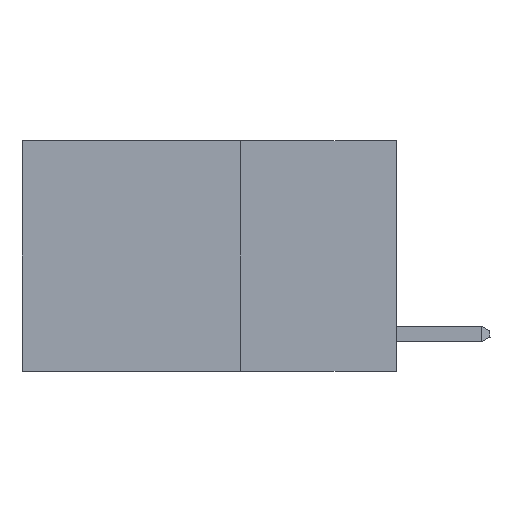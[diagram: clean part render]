
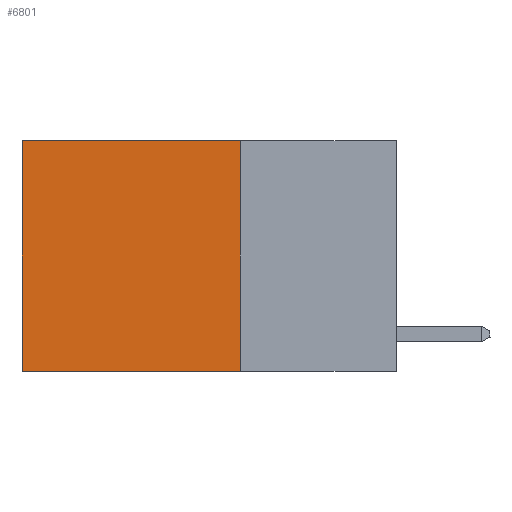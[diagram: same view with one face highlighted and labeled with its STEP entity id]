
A CAD part, left-side view. The second image highlights one B-rep face of the part: STEP entity #6801.
In plain terms, the highlighted planar face has unit normal (-1, 0, 0).
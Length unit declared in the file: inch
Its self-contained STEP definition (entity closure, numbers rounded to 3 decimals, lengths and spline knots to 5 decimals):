
#1606 = DIRECTION ( 'NONE',  ( 0., 0., -1. ) ) ;
#2007 = ORIENTED_EDGE ( 'NONE', *, *, #9132, .T. ) ;
#2171 = VECTOR ( 'NONE', #1606, 39.37008 ) ;
#2931 = VECTOR ( 'NONE', #3925, 39.37008 ) ;
#3206 = VERTEX_POINT ( 'NONE', #3511 ) ;
#3344 = EDGE_LOOP ( 'NONE', ( #2007, #4901, #6341, #5074 ) ) ;
#3403 = CARTESIAN_POINT ( 'NONE',  ( 0.2625, 0.25, -0.37 ) ) ;
#3511 = CARTESIAN_POINT ( 'NONE',  ( 0.2625, 0.25, 0. ) ) ;
#3925 = DIRECTION ( 'NONE',  ( 0., 0., -1. ) ) ;
#4595 = LINE ( 'NONE', #14483, #11349 ) ;
#4901 = ORIENTED_EDGE ( 'NONE', *, *, #15257, .F. ) ;
#5074 = ORIENTED_EDGE ( 'NONE', *, *, #5705, .T. ) ;
#5705 = EDGE_CURVE ( 'NONE', #3206, #10003, #4595, .T. ) ;
#6341 = ORIENTED_EDGE ( 'NONE', *, *, #10054, .F. ) ;
#6472 = CARTESIAN_POINT ( 'NONE',  ( 0.2625, 0.6, 0. ) ) ;
#6613 = VERTEX_POINT ( 'NONE', #13320 ) ;
#6801 = ADVANCED_FACE ( 'NONE', ( #15314 ), #8146, .F. ) ;
#6982 = DIRECTION ( 'NONE',  ( 0., 1., 0. ) ) ;
#7580 = LINE ( 'NONE', #8777, #2171 ) ;
#7983 = DIRECTION ( 'NONE',  ( 0., 0., -1. ) ) ;
#8146 = PLANE ( 'NONE',  #10819 ) ;
#8777 = CARTESIAN_POINT ( 'NONE',  ( 0.2625, 0.6, 0. ) ) ;
#9071 = CARTESIAN_POINT ( 'NONE',  ( 0.2625, 0.25, -0.37 ) ) ;
#9132 = EDGE_CURVE ( 'NONE', #10003, #6613, #7580, .T. ) ;
#9181 = DIRECTION ( 'NONE',  ( 0., 1., 0. ) ) ;
#9740 = VERTEX_POINT ( 'NONE', #9071 ) ;
#10003 = VERTEX_POINT ( 'NONE', #6472 ) ;
#10015 = LINE ( 'NONE', #14932, #2931 ) ;
#10054 = EDGE_CURVE ( 'NONE', #3206, #9740, #10015, .T. ) ;
#10480 = DIRECTION ( 'NONE',  ( 1., 0., 0. ) ) ;
#10710 = VECTOR ( 'NONE', #6982, 39.37008 ) ;
#10819 = AXIS2_PLACEMENT_3D ( 'NONE', #11779, #10480, #7983 ) ;
#11349 = VECTOR ( 'NONE', #9181, 39.37008 ) ;
#11779 = CARTESIAN_POINT ( 'NONE',  ( 0.2625, 0.25, 0. ) ) ;
#13320 = CARTESIAN_POINT ( 'NONE',  ( 0.2625, 0.6, -0.37 ) ) ;
#14399 = LINE ( 'NONE', #3403, #10710 ) ;
#14483 = CARTESIAN_POINT ( 'NONE',  ( 0.2625, 0.25, 0. ) ) ;
#14932 = CARTESIAN_POINT ( 'NONE',  ( 0.2625, 0.25, 0. ) ) ;
#15257 = EDGE_CURVE ( 'NONE', #9740, #6613, #14399, .T. ) ;
#15314 = FACE_OUTER_BOUND ( 'NONE', #3344, .T. ) ;
